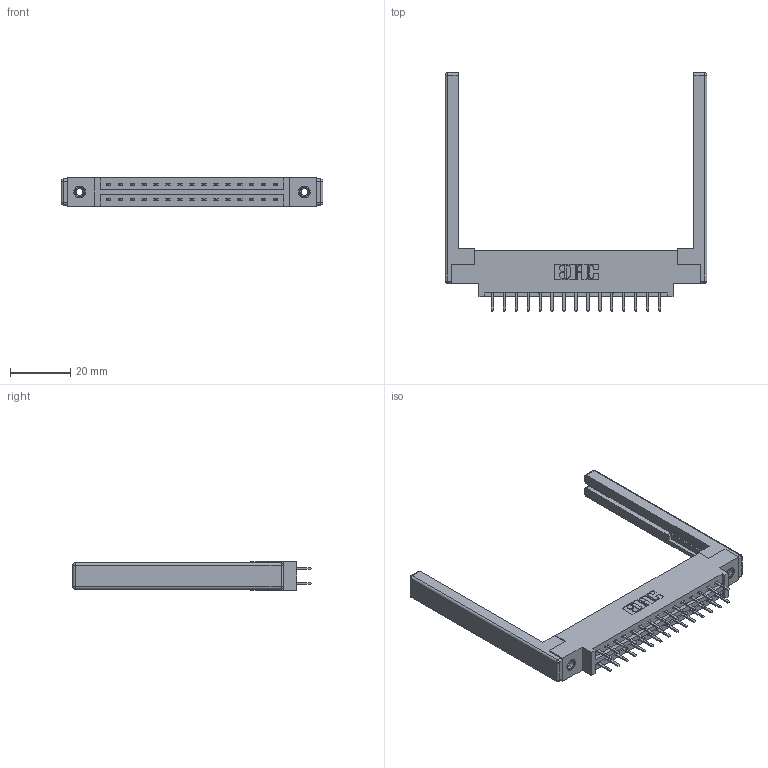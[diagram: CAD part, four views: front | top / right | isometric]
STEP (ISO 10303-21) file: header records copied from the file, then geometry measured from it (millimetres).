
FILE_DESCRIPTION (( 'STEP AP203' ), '1' );
FILE_NAME ('337-030-520-868.STEP', '2019-10-10T23:26:10', ( '' ), ( '' ), 'SwSTEP 2.0', 'SolidWorks 2016', '' );
FILE_SCHEMA (( 'CONFIG_CONTROL_DESIGN' ));
Length unit declared in the file: inch
Products named in the file (5): 337-030-520-868; 307-220-068; 337 Part_0.170 Offset - 0.156 Dia-TI; 345-292-001_345-293-120; 345-250-001_345-250-001-102
Assembly tree (35 placements, depth 2):
  337-030-520-868
    337 Part_0.170 Offset - 0.156 Dia-TI
    345-292-001_345-293-120  x30
    345-250-001_345-250-001-102  x2
    307-220-068  x2
Bounding box: 86.87 x 79.08 x 9.4 mm (x, y, z)
Volume: 13049.5 mm3; surface area: 13637.8 mm2
Topology: 35 solids, 35 shells, 2012 faces, 5783 edges, 3754 vertices
Faces by surface type: plane 1362, cylinder 626, cone 12, sphere 8, torus 4
Entity records: 18128 total; most frequent: CARTESIAN_POINT 3055, ORIENTED_EDGE 2968, DIRECTION 2706, EDGE_CURVE 1484, VECTOR 1302, LINE 1302, VERTEX_POINT 978, AXIS2_PLACEMENT_3D 702
